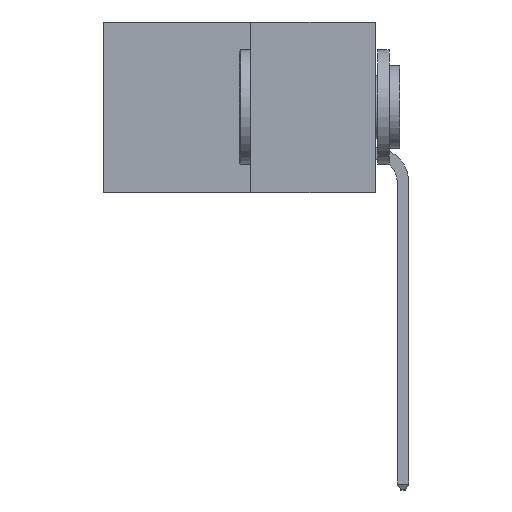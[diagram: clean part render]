
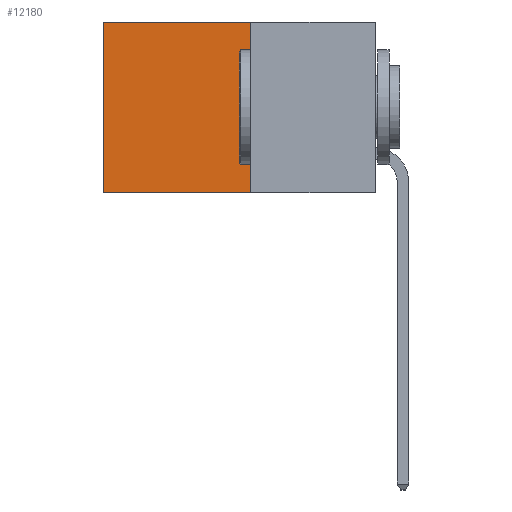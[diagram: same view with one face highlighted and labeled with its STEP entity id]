
A CAD part, left-side view. The second image highlights one B-rep face of the part: STEP entity #12180.
In plain terms, the highlighted planar face has unit normal (-1, 0, 0).
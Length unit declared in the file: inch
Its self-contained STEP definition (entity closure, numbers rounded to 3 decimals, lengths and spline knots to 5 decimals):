
#450 = LINE ( 'NONE', #7962, #2204 ) ;
#747 = CARTESIAN_POINT ( 'NONE',  ( 0.277, 0.27, -0.37 ) ) ;
#1193 = VERTEX_POINT ( 'NONE', #2726 ) ;
#1648 = DIRECTION ( 'NONE',  ( 0., 0., -1. ) ) ;
#1926 = EDGE_CURVE ( 'NONE', #7122, #1193, #3930, .T. ) ;
#2064 = CARTESIAN_POINT ( 'NONE',  ( 0.277, 0.59, -0.37 ) ) ;
#2204 = VECTOR ( 'NONE', #1648, 39.37008 ) ;
#2285 = CARTESIAN_POINT ( 'NONE',  ( 0.277, 0.27, -0.37 ) ) ;
#2571 = DIRECTION ( 'NONE',  ( 0., 1., 0. ) ) ;
#2726 = CARTESIAN_POINT ( 'NONE',  ( 0.277, 0.59, 0. ) ) ;
#3177 = VECTOR ( 'NONE', #14430, 39.37008 ) ;
#3231 = EDGE_LOOP ( 'NONE', ( #11380, #14653, #15024, #5437 ) ) ;
#3305 = VERTEX_POINT ( 'NONE', #2064 ) ;
#3930 = LINE ( 'NONE', #8326, #9459 ) ;
#4397 = CARTESIAN_POINT ( 'NONE',  ( 0.277, 0.27, -0.37 ) ) ;
#4841 = CARTESIAN_POINT ( 'NONE',  ( 0.277, 0.27, 0. ) ) ;
#5437 = ORIENTED_EDGE ( 'NONE', *, *, #1926, .T. ) ;
#6431 = FACE_OUTER_BOUND ( 'NONE', #3231, .T. ) ;
#7122 = VERTEX_POINT ( 'NONE', #4841 ) ;
#7306 = EDGE_CURVE ( 'NONE', #7122, #9738, #14621, .T. ) ;
#7779 = DIRECTION ( 'NONE',  ( 0., 0., -1. ) ) ;
#7962 = CARTESIAN_POINT ( 'NONE',  ( 0.277, 0.59, -0.37 ) ) ;
#8182 = AXIS2_PLACEMENT_3D ( 'NONE', #2285, #16014, #8651 ) ;
#8326 = CARTESIAN_POINT ( 'NONE',  ( 0.277, 0.27, 0. ) ) ;
#8353 = EDGE_CURVE ( 'NONE', #1193, #3305, #450, .T. ) ;
#8651 = DIRECTION ( 'NONE',  ( 0., 0., -1. ) ) ;
#9041 = CARTESIAN_POINT ( 'NONE',  ( 0.277, 0.27, -0.37 ) ) ;
#9459 = VECTOR ( 'NONE', #2571, 39.37008 ) ;
#9738 = VERTEX_POINT ( 'NONE', #747 ) ;
#10940 = VECTOR ( 'NONE', #7779, 39.37008 ) ;
#11380 = ORIENTED_EDGE ( 'NONE', *, *, #8353, .T. ) ;
#12180 = ADVANCED_FACE ( 'NONE', ( #6431 ), #12371, .F. ) ;
#12371 = PLANE ( 'NONE',  #8182 ) ;
#14430 = DIRECTION ( 'NONE',  ( 0., 1., 0. ) ) ;
#14621 = LINE ( 'NONE', #9041, #10940 ) ;
#14653 = ORIENTED_EDGE ( 'NONE', *, *, #15648, .F. ) ;
#15024 = ORIENTED_EDGE ( 'NONE', *, *, #7306, .F. ) ;
#15648 = EDGE_CURVE ( 'NONE', #9738, #3305, #15663, .T. ) ;
#15663 = LINE ( 'NONE', #4397, #3177 ) ;
#16014 = DIRECTION ( 'NONE',  ( 1., 0., 0. ) ) ;
